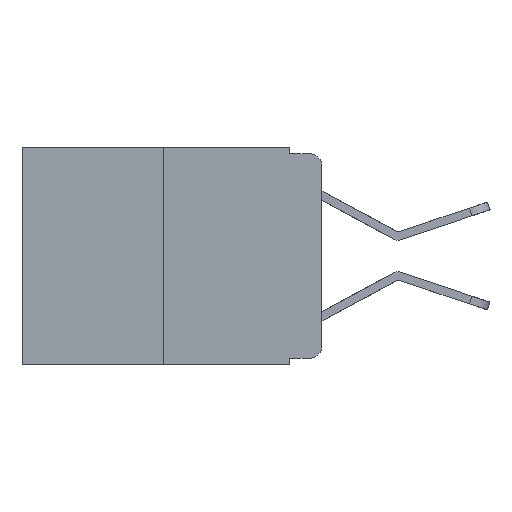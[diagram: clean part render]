
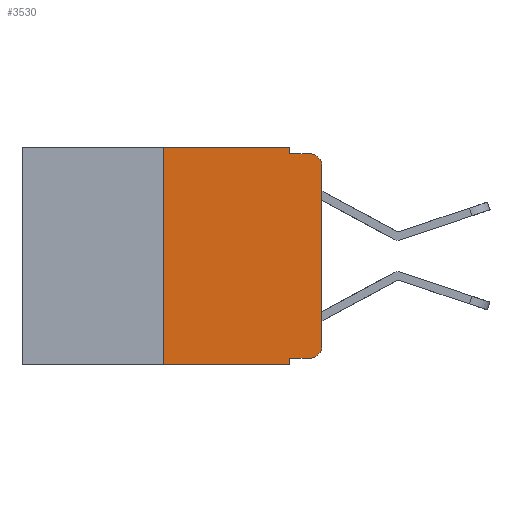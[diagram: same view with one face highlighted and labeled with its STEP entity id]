
A CAD part, left-side view. The second image highlights one B-rep face of the part: STEP entity #3530.
In plain terms, the highlighted planar face has unit normal (-1, 0, 0).
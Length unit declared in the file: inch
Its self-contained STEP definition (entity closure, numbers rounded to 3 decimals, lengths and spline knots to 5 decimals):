
#38 = EDGE_CURVE ( 'NONE', #6395, #7262, #8843, .T. ) ;
#56 = LINE ( 'NONE', #9984, #15603 ) ;
#221 = DIRECTION ( 'NONE',  ( 0., -1., 0. ) ) ;
#225 = ORIENTED_EDGE ( 'NONE', *, *, #17934, .T. ) ;
#612 = VERTEX_POINT ( 'NONE', #12700 ) ;
#676 = DIRECTION ( 'NONE',  ( 0., -1., 0. ) ) ;
#1232 = ORIENTED_EDGE ( 'NONE', *, *, #2795, .F. ) ;
#1327 = DIRECTION ( 'NONE',  ( 0., 0., -1. ) ) ;
#1430 = PLANE ( 'NONE',  #3320 ) ;
#1451 = DIRECTION ( 'NONE',  ( 0., 0., -1. ) ) ;
#1485 = VECTOR ( 'NONE', #6890, 39.37008 ) ;
#1550 = DIRECTION ( 'NONE',  ( 0., 0., -1. ) ) ;
#2119 = CARTESIAN_POINT ( 'NONE',  ( 0., 0.051, -0.333 ) ) ;
#2144 = VERTEX_POINT ( 'NONE', #5370 ) ;
#2559 = CARTESIAN_POINT ( 'NONE',  ( 0., 0.051, 0. ) ) ;
#2763 = DIRECTION ( 'NONE',  ( 1., 0., 0. ) ) ;
#2795 = EDGE_CURVE ( 'NONE', #6395, #14606, #10269, .T. ) ;
#3103 = ORIENTED_EDGE ( 'NONE', *, *, #10722, .T. ) ;
#3320 = AXIS2_PLACEMENT_3D ( 'NONE', #17012, #2763, #1550 ) ;
#3381 = LINE ( 'NONE', #2119, #17522 ) ;
#3530 = ADVANCED_FACE ( 'NONE', ( #12874 ), #1430, .F. ) ;
#3680 = AXIS2_PLACEMENT_3D ( 'NONE', #18263, #9860, #1327 ) ;
#4049 = DIRECTION ( 'NONE',  ( 0., 0., 1. ) ) ;
#4230 = ORIENTED_EDGE ( 'NONE', *, *, #7564, .F. ) ;
#4538 = DIRECTION ( 'NONE',  ( 0., 0., 1. ) ) ;
#4611 = VERTEX_POINT ( 'NONE', #8983 ) ;
#4789 = CARTESIAN_POINT ( 'NONE',  ( 0., 0.473, -0.343 ) ) ;
#5016 = VECTOR ( 'NONE', #221, 39.37008 ) ;
#5159 = VERTEX_POINT ( 'NONE', #10274 ) ;
#5370 = CARTESIAN_POINT ( 'NONE',  ( 0., 0.051, -0.333 ) ) ;
#5559 = CARTESIAN_POINT ( 'NONE',  ( 0., 0.051, -0.01 ) ) ;
#5783 = DIRECTION ( 'NONE',  ( -1., 0., 0. ) ) ;
#6023 = VECTOR ( 'NONE', #4049, 39.37008 ) ;
#6346 = DIRECTION ( 'NONE',  ( 0., -1., 0. ) ) ;
#6395 = VERTEX_POINT ( 'NONE', #7413 ) ;
#6833 = AXIS2_PLACEMENT_3D ( 'NONE', #14267, #5783, #15689 ) ;
#6890 = DIRECTION ( 'NONE',  ( 0., -1., 0. ) ) ;
#7262 = VERTEX_POINT ( 'NONE', #7813 ) ;
#7413 = CARTESIAN_POINT ( 'NONE',  ( 0., 0.25, -0.343 ) ) ;
#7564 = EDGE_CURVE ( 'NONE', #612, #11992, #56, .T. ) ;
#7813 = CARTESIAN_POINT ( 'NONE',  ( 0., 0.051, -0.343 ) ) ;
#7970 = CARTESIAN_POINT ( 'NONE',  ( 0., 0.25, 0. ) ) ;
#8198 = VECTOR ( 'NONE', #6346, 39.37008 ) ;
#8215 = CARTESIAN_POINT ( 'NONE',  ( 0., 0.02, -0.333 ) ) ;
#8465 = CARTESIAN_POINT ( 'NONE',  ( 0., 0., -0.313 ) ) ;
#8613 = LINE ( 'NONE', #15347, #1485 ) ;
#8843 = LINE ( 'NONE', #4789, #5016 ) ;
#8983 = CARTESIAN_POINT ( 'NONE',  ( 0., 0.02, -0.01 ) ) ;
#9439 = CARTESIAN_POINT ( 'NONE',  ( 0., 0.25, 0. ) ) ;
#9860 = DIRECTION ( 'NONE',  ( -1., 0., 0. ) ) ;
#9984 = CARTESIAN_POINT ( 'NONE',  ( 0., 0.051, 0. ) ) ;
#10175 = ORIENTED_EDGE ( 'NONE', *, *, #18277, .F. ) ;
#10269 = LINE ( 'NONE', #7970, #6023 ) ;
#10274 = CARTESIAN_POINT ( 'NONE',  ( 0., 0., -0.03 ) ) ;
#10396 = EDGE_CURVE ( 'NONE', #11992, #4611, #11966, .T. ) ;
#10430 = ORIENTED_EDGE ( 'NONE', *, *, #11254, .F. ) ;
#10444 = ORIENTED_EDGE ( 'NONE', *, *, #38, .T. ) ;
#10576 = LINE ( 'NONE', #2559, #13879 ) ;
#10722 = EDGE_CURVE ( 'NONE', #18275, #11336, #10825, .T. ) ;
#10821 = ORIENTED_EDGE ( 'NONE', *, *, #10396, .F. ) ;
#10825 = CIRCLE ( 'NONE', #6833, 0.02 ) ;
#11254 = EDGE_CURVE ( 'NONE', #14606, #612, #8613, .T. ) ;
#11336 = VERTEX_POINT ( 'NONE', #8465 ) ;
#11966 = LINE ( 'NONE', #17661, #8198 ) ;
#11992 = VERTEX_POINT ( 'NONE', #5559 ) ;
#12700 = CARTESIAN_POINT ( 'NONE',  ( 0., 0.051, 0. ) ) ;
#12714 = CIRCLE ( 'NONE', #3680, 0.02 ) ;
#12874 = FACE_OUTER_BOUND ( 'NONE', #17925, .T. ) ;
#13867 = DIRECTION ( 'NONE',  ( 0., 0., -1. ) ) ;
#13879 = VECTOR ( 'NONE', #13867, 39.37008 ) ;
#14105 = ORIENTED_EDGE ( 'NONE', *, *, #15478, .T. ) ;
#14267 = CARTESIAN_POINT ( 'NONE',  ( 0., 0.02, -0.313 ) ) ;
#14459 = CARTESIAN_POINT ( 'NONE',  ( 0., 0., 0. ) ) ;
#14606 = VERTEX_POINT ( 'NONE', #9439 ) ;
#15116 = EDGE_CURVE ( 'NONE', #5159, #4611, #12714, .T. ) ;
#15347 = CARTESIAN_POINT ( 'NONE',  ( 0., 0.473, 0. ) ) ;
#15478 = EDGE_CURVE ( 'NONE', #2144, #18275, #3381, .T. ) ;
#15603 = VECTOR ( 'NONE', #1451, 39.37008 ) ;
#15689 = DIRECTION ( 'NONE',  ( 0., 0., -1. ) ) ;
#16339 = VECTOR ( 'NONE', #4538, 39.37008 ) ;
#16355 = ORIENTED_EDGE ( 'NONE', *, *, #15116, .T. ) ;
#17012 = CARTESIAN_POINT ( 'NONE',  ( 0., 0.473, 0. ) ) ;
#17215 = LINE ( 'NONE', #14459, #16339 ) ;
#17522 = VECTOR ( 'NONE', #676, 39.37008 ) ;
#17661 = CARTESIAN_POINT ( 'NONE',  ( 0., 0.051, -0.01 ) ) ;
#17925 = EDGE_LOOP ( 'NONE', ( #225, #16355, #10821, #4230, #10430, #1232, #10444, #10175, #14105, #3103 ) ) ;
#17934 = EDGE_CURVE ( 'NONE', #11336, #5159, #17215, .T. ) ;
#18263 = CARTESIAN_POINT ( 'NONE',  ( 0., 0.02, -0.03 ) ) ;
#18275 = VERTEX_POINT ( 'NONE', #8215 ) ;
#18277 = EDGE_CURVE ( 'NONE', #2144, #7262, #10576, .T. ) ;
